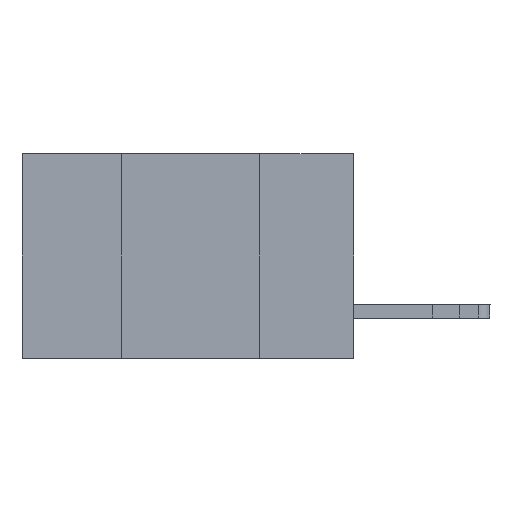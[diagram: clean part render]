
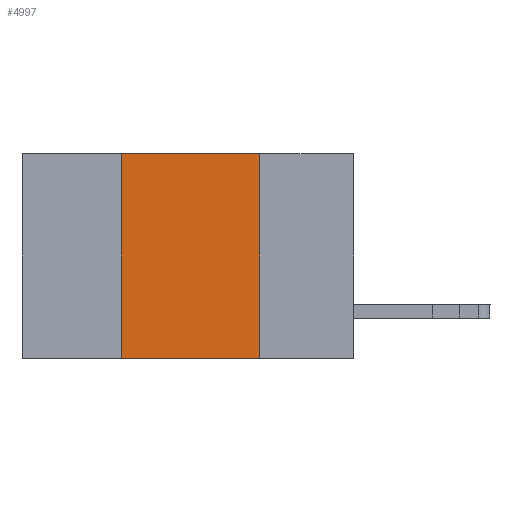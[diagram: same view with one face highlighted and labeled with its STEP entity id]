
A CAD part, left-side view. The second image highlights one B-rep face of the part: STEP entity #4997.
In plain terms, the highlighted planar face has unit normal (-1, 0, 0).
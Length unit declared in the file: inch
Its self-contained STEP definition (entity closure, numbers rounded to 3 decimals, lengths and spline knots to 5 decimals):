
#20 = VERTEX_POINT ( 'NONE', #7858 ) ;
#1081 = AXIS2_PLACEMENT_3D ( 'NONE', #7555, #11616, #15662 ) ;
#1405 = VERTEX_POINT ( 'NONE', #16071 ) ;
#3013 = EDGE_CURVE ( 'NONE', #5306, #20, #5362, .T. ) ;
#3032 = VECTOR ( 'NONE', #3640, 39.37008 ) ;
#3388 = CARTESIAN_POINT ( 'NONE',  ( 0., 0.17, 0. ) ) ;
#3640 = DIRECTION ( 'NONE',  ( 0., 0., -1. ) ) ;
#3952 = EDGE_CURVE ( 'NONE', #1405, #14763, #16490, .T. ) ;
#4011 = ORIENTED_EDGE ( 'NONE', *, *, #3952, .F. ) ;
#4997 = ADVANCED_FACE ( 'NONE', ( #12237 ), #14418, .F. ) ;
#5306 = VERTEX_POINT ( 'NONE', #5833 ) ;
#5362 = LINE ( 'NONE', #3388, #3032 ) ;
#5833 = CARTESIAN_POINT ( 'NONE',  ( 0., 0.17, 0. ) ) ;
#6015 = ORIENTED_EDGE ( 'NONE', *, *, #9225, .T. ) ;
#7555 = CARTESIAN_POINT ( 'NONE',  ( 0., 0.6, 0. ) ) ;
#7817 = CARTESIAN_POINT ( 'NONE',  ( 0., 0.42, 0. ) ) ;
#7858 = CARTESIAN_POINT ( 'NONE',  ( 0., 0.17, -0.37 ) ) ;
#8556 = ORIENTED_EDGE ( 'NONE', *, *, #3013, .F. ) ;
#9201 = CARTESIAN_POINT ( 'NONE',  ( 0., 0.6, 0. ) ) ;
#9225 = EDGE_CURVE ( 'NONE', #1405, #20, #11694, .T. ) ;
#10496 = ORIENTED_EDGE ( 'NONE', *, *, #13546, .F. ) ;
#11616 = DIRECTION ( 'NONE',  ( 1., 0., 0. ) ) ;
#11694 = LINE ( 'NONE', #16400, #12749 ) ;
#12237 = FACE_OUTER_BOUND ( 'NONE', #13343, .T. ) ;
#12284 = VECTOR ( 'NONE', #17342, 39.37008 ) ;
#12749 = VECTOR ( 'NONE', #16520, 39.37008 ) ;
#13262 = VECTOR ( 'NONE', #14771, 39.37008 ) ;
#13343 = EDGE_LOOP ( 'NONE', ( #8556, #10496, #4011, #6015 ) ) ;
#13546 = EDGE_CURVE ( 'NONE', #14763, #5306, #14280, .T. ) ;
#14280 = LINE ( 'NONE', #9201, #13262 ) ;
#14418 = PLANE ( 'NONE',  #1081 ) ;
#14763 = VERTEX_POINT ( 'NONE', #7817 ) ;
#14771 = DIRECTION ( 'NONE',  ( 0., -1., 0. ) ) ;
#15662 = DIRECTION ( 'NONE',  ( 0., 0., -1. ) ) ;
#15975 = CARTESIAN_POINT ( 'NONE',  ( 0., 0.42, 0. ) ) ;
#16071 = CARTESIAN_POINT ( 'NONE',  ( 0., 0.42, -0.37 ) ) ;
#16400 = CARTESIAN_POINT ( 'NONE',  ( 0., 0.6, -0.37 ) ) ;
#16490 = LINE ( 'NONE', #15975, #12284 ) ;
#16520 = DIRECTION ( 'NONE',  ( 0., -1., 0. ) ) ;
#17342 = DIRECTION ( 'NONE',  ( 0., 0., 1. ) ) ;
